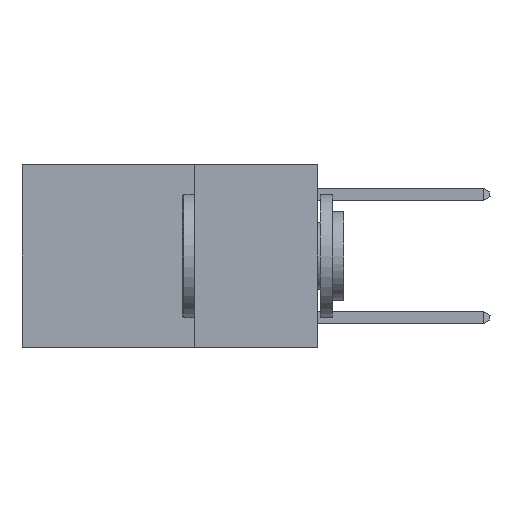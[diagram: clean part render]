
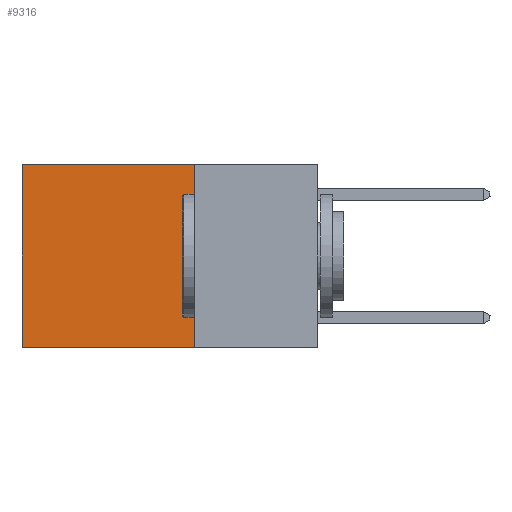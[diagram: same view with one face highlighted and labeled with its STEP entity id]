
A CAD part, left-side view. The second image highlights one B-rep face of the part: STEP entity #9316.
In plain terms, the highlighted planar face has unit normal (-1, 0, 0).
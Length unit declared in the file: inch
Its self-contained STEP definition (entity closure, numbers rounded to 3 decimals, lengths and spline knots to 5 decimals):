
#153 = VECTOR ( 'NONE', #3546, 39.37008 ) ;
#1385 = LINE ( 'NONE', #11781, #10733 ) ;
#1969 = LINE ( 'NONE', #3321, #3667 ) ;
#2042 = CARTESIAN_POINT ( 'NONE',  ( 0.2625, 0.25, 0. ) ) ;
#2584 = DIRECTION ( 'NONE',  ( 1., 0., 0. ) ) ;
#2714 = CARTESIAN_POINT ( 'NONE',  ( 0.2625, 0.6, 0. ) ) ;
#3321 = CARTESIAN_POINT ( 'NONE',  ( 0.2625, 0.25, 0. ) ) ;
#3546 = DIRECTION ( 'NONE',  ( 0., 0., -1. ) ) ;
#3667 = VECTOR ( 'NONE', #7175, 39.37008 ) ;
#4333 = EDGE_CURVE ( 'NONE', #7021, #13495, #1969, .T. ) ;
#4718 = CARTESIAN_POINT ( 'NONE',  ( 0.2625, 0.25, 0. ) ) ;
#5277 = LINE ( 'NONE', #7466, #9782 ) ;
#5280 = CARTESIAN_POINT ( 'NONE',  ( 0.2625, 0.6, 0. ) ) ;
#5497 = DIRECTION ( 'NONE',  ( 0., 0., -1. ) ) ;
#6482 = EDGE_CURVE ( 'NONE', #10449, #7810, #5277, .T. ) ;
#6491 = EDGE_LOOP ( 'NONE', ( #12822, #8257, #7441, #10692 ) ) ;
#7021 = VERTEX_POINT ( 'NONE', #2042 ) ;
#7175 = DIRECTION ( 'NONE',  ( 0., 1., 0. ) ) ;
#7337 = CARTESIAN_POINT ( 'NONE',  ( 0.2625, 0.25, -0.37 ) ) ;
#7441 = ORIENTED_EDGE ( 'NONE', *, *, #13221, .F. ) ;
#7452 = AXIS2_PLACEMENT_3D ( 'NONE', #4718, #2584, #12016 ) ;
#7466 = CARTESIAN_POINT ( 'NONE',  ( 0.2625, 0.25, -0.37 ) ) ;
#7810 = VERTEX_POINT ( 'NONE', #9481 ) ;
#7984 = EDGE_CURVE ( 'NONE', #13495, #7810, #10010, .T. ) ;
#8257 = ORIENTED_EDGE ( 'NONE', *, *, #6482, .F. ) ;
#9316 = ADVANCED_FACE ( 'NONE', ( #13023 ), #10970, .F. ) ;
#9481 = CARTESIAN_POINT ( 'NONE',  ( 0.2625, 0.6, -0.37 ) ) ;
#9782 = VECTOR ( 'NONE', #12574, 39.37008 ) ;
#10010 = LINE ( 'NONE', #2714, #153 ) ;
#10449 = VERTEX_POINT ( 'NONE', #7337 ) ;
#10692 = ORIENTED_EDGE ( 'NONE', *, *, #4333, .T. ) ;
#10733 = VECTOR ( 'NONE', #5497, 39.37008 ) ;
#10970 = PLANE ( 'NONE',  #7452 ) ;
#11781 = CARTESIAN_POINT ( 'NONE',  ( 0.2625, 0.25, 0. ) ) ;
#12016 = DIRECTION ( 'NONE',  ( 0., 0., -1. ) ) ;
#12574 = DIRECTION ( 'NONE',  ( 0., 1., 0. ) ) ;
#12822 = ORIENTED_EDGE ( 'NONE', *, *, #7984, .T. ) ;
#13023 = FACE_OUTER_BOUND ( 'NONE', #6491, .T. ) ;
#13221 = EDGE_CURVE ( 'NONE', #7021, #10449, #1385, .T. ) ;
#13495 = VERTEX_POINT ( 'NONE', #5280 ) ;
